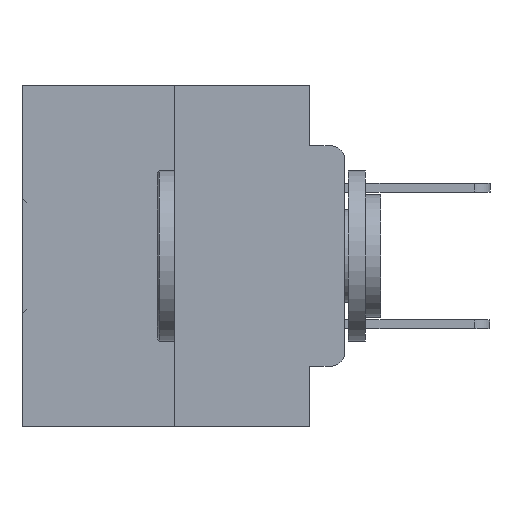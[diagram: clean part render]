
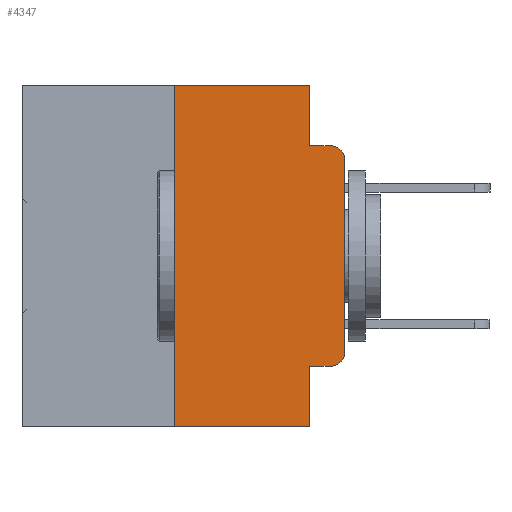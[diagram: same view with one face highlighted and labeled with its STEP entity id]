
A CAD part, left-side view. The second image highlights one B-rep face of the part: STEP entity #4347.
In plain terms, the highlighted planar face has unit normal (-1, 0, 0).
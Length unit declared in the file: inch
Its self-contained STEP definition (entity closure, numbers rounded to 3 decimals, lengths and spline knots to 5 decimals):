
#99 = DIRECTION ( 'NONE',  ( 0., 0., -1. ) ) ;
#233 = VECTOR ( 'NONE', #99, 39.37008 ) ;
#1491 = EDGE_CURVE ( 'NONE', #12993, #7114, #13435, .T. ) ;
#1704 = ORIENTED_EDGE ( 'NONE', *, *, #12898, .F. ) ;
#3049 = LINE ( 'NONE', #9296, #9447 ) ;
#3282 = VECTOR ( 'NONE', #22996, 39.37008 ) ;
#3565 = AXIS2_PLACEMENT_3D ( 'NONE', #24149, #8043, #26870 ) ;
#3890 = VERTEX_POINT ( 'NONE', #7036 ) ;
#4078 = VECTOR ( 'NONE', #24456, 39.37008 ) ;
#4347 = ADVANCED_FACE ( 'NONE', ( #9129 ), #5259, .F. ) ;
#4535 = CARTESIAN_POINT ( 'NONE',  ( 0., 0.051, -0.5 ) ) ;
#5165 = ORIENTED_EDGE ( 'NONE', *, *, #16939, .F. ) ;
#5259 = PLANE ( 'NONE',  #25451 ) ;
#5618 = CARTESIAN_POINT ( 'NONE',  ( 0., 0.051, -0.0885 ) ) ;
#5847 = EDGE_CURVE ( 'NONE', #12053, #12993, #3049, .T. ) ;
#6216 = AXIS2_PLACEMENT_3D ( 'NONE', #25947, #25535, #26237 ) ;
#6814 = ORIENTED_EDGE ( 'NONE', *, *, #12018, .F. ) ;
#7036 = CARTESIAN_POINT ( 'NONE',  ( 0., 0.051, 0. ) ) ;
#7114 = VERTEX_POINT ( 'NONE', #25069 ) ;
#7149 = VECTOR ( 'NONE', #28899, 39.37008 ) ;
#7513 = CARTESIAN_POINT ( 'NONE',  ( 0., 0.25, 0. ) ) ;
#7884 = LINE ( 'NONE', #29065, #21393 ) ;
#7937 = EDGE_LOOP ( 'NONE', ( #29117, #20766, #1704, #5165, #34584, #15768, #26241, #6814, #9366, #34133 ) ) ;
#7986 = EDGE_CURVE ( 'NONE', #28343, #34374, #14389, .T. ) ;
#8023 = VECTOR ( 'NONE', #30246, 39.37008 ) ;
#8043 = DIRECTION ( 'NONE',  ( -1., 0., 0. ) ) ;
#8530 = VERTEX_POINT ( 'NONE', #15181 ) ;
#9129 = FACE_OUTER_BOUND ( 'NONE', #7937, .T. ) ;
#9296 = CARTESIAN_POINT ( 'NONE',  ( 0., 0.051, -0.4115 ) ) ;
#9366 = ORIENTED_EDGE ( 'NONE', *, *, #5847, .T. ) ;
#9447 = VECTOR ( 'NONE', #12061, 39.37008 ) ;
#9918 = CARTESIAN_POINT ( 'NONE',  ( 0., 0.051, -0.0885 ) ) ;
#10737 = DIRECTION ( 'NONE',  ( 1., 0., 0. ) ) ;
#10881 = EDGE_CURVE ( 'NONE', #28343, #8530, #26163, .T. ) ;
#12018 = EDGE_CURVE ( 'NONE', #12053, #34374, #31934, .T. ) ;
#12053 = VERTEX_POINT ( 'NONE', #23107 ) ;
#12061 = DIRECTION ( 'NONE',  ( 0., -1., 0. ) ) ;
#12898 = EDGE_CURVE ( 'NONE', #16657, #27904, #24742, .T. ) ;
#12993 = VERTEX_POINT ( 'NONE', #22128 ) ;
#13046 = DIRECTION ( 'NONE',  ( 0., -1., 0. ) ) ;
#13435 = CIRCLE ( 'NONE', #6216, 0.02 ) ;
#13489 = EDGE_CURVE ( 'NONE', #8530, #3890, #7884, .T. ) ;
#14389 = LINE ( 'NONE', #34144, #7149 ) ;
#15181 = CARTESIAN_POINT ( 'NONE',  ( 0., 0.25, 0. ) ) ;
#15367 = EDGE_CURVE ( 'NONE', #18500, #27904, #21261, .T. ) ;
#15487 = CARTESIAN_POINT ( 'NONE',  ( 0., 0., -0.1085 ) ) ;
#15768 = ORIENTED_EDGE ( 'NONE', *, *, #10881, .F. ) ;
#16657 = VERTEX_POINT ( 'NONE', #9918 ) ;
#16939 = EDGE_CURVE ( 'NONE', #3890, #16657, #21861, .T. ) ;
#18500 = VERTEX_POINT ( 'NONE', #15487 ) ;
#19077 = CARTESIAN_POINT ( 'NONE',  ( 0., 0.051, 0. ) ) ;
#19486 = CARTESIAN_POINT ( 'NONE',  ( 0., 0., 0. ) ) ;
#20766 = ORIENTED_EDGE ( 'NONE', *, *, #15367, .T. ) ;
#21261 = CIRCLE ( 'NONE', #3565, 0.02 ) ;
#21393 = VECTOR ( 'NONE', #13046, 39.37008 ) ;
#21861 = LINE ( 'NONE', #19077, #233 ) ;
#22128 = CARTESIAN_POINT ( 'NONE',  ( 0., 0.02, -0.4115 ) ) ;
#22996 = DIRECTION ( 'NONE',  ( 0., 0., -1. ) ) ;
#23107 = CARTESIAN_POINT ( 'NONE',  ( 0., 0.051, -0.4115 ) ) ;
#23202 = EDGE_CURVE ( 'NONE', #7114, #18500, #29464, .T. ) ;
#24149 = CARTESIAN_POINT ( 'NONE',  ( 0., 0.02, -0.1085 ) ) ;
#24456 = DIRECTION ( 'NONE',  ( 0., -1., 0. ) ) ;
#24742 = LINE ( 'NONE', #5618, #4078 ) ;
#25069 = CARTESIAN_POINT ( 'NONE',  ( 0., 0., -0.3915 ) ) ;
#25451 = AXIS2_PLACEMENT_3D ( 'NONE', #34741, #10737, #29478 ) ;
#25535 = DIRECTION ( 'NONE',  ( -1., 0., 0. ) ) ;
#25947 = CARTESIAN_POINT ( 'NONE',  ( 0., 0.02, -0.3915 ) ) ;
#26163 = LINE ( 'NONE', #7513, #32441 ) ;
#26237 = DIRECTION ( 'NONE',  ( 0., 0., -1. ) ) ;
#26241 = ORIENTED_EDGE ( 'NONE', *, *, #7986, .T. ) ;
#26870 = DIRECTION ( 'NONE',  ( 0., 0., -1. ) ) ;
#27904 = VERTEX_POINT ( 'NONE', #34017 ) ;
#28343 = VERTEX_POINT ( 'NONE', #30949 ) ;
#28899 = DIRECTION ( 'NONE',  ( 0., -1., 0. ) ) ;
#29065 = CARTESIAN_POINT ( 'NONE',  ( 0., 0.473, 0. ) ) ;
#29117 = ORIENTED_EDGE ( 'NONE', *, *, #23202, .T. ) ;
#29464 = LINE ( 'NONE', #19486, #8023 ) ;
#29478 = DIRECTION ( 'NONE',  ( 0., 0., -1. ) ) ;
#30246 = DIRECTION ( 'NONE',  ( 0., 0., 1. ) ) ;
#30949 = CARTESIAN_POINT ( 'NONE',  ( 0., 0.25, -0.5 ) ) ;
#31710 = DIRECTION ( 'NONE',  ( 0., 0., 1. ) ) ;
#31934 = LINE ( 'NONE', #33628, #3282 ) ;
#32441 = VECTOR ( 'NONE', #31710, 39.37008 ) ;
#33628 = CARTESIAN_POINT ( 'NONE',  ( 0., 0.051, 0. ) ) ;
#34017 = CARTESIAN_POINT ( 'NONE',  ( 0., 0.02, -0.0885 ) ) ;
#34133 = ORIENTED_EDGE ( 'NONE', *, *, #1491, .T. ) ;
#34144 = CARTESIAN_POINT ( 'NONE',  ( 0., 0.473, -0.5 ) ) ;
#34374 = VERTEX_POINT ( 'NONE', #4535 ) ;
#34584 = ORIENTED_EDGE ( 'NONE', *, *, #13489, .F. ) ;
#34741 = CARTESIAN_POINT ( 'NONE',  ( 0., 0.473, 0. ) ) ;
